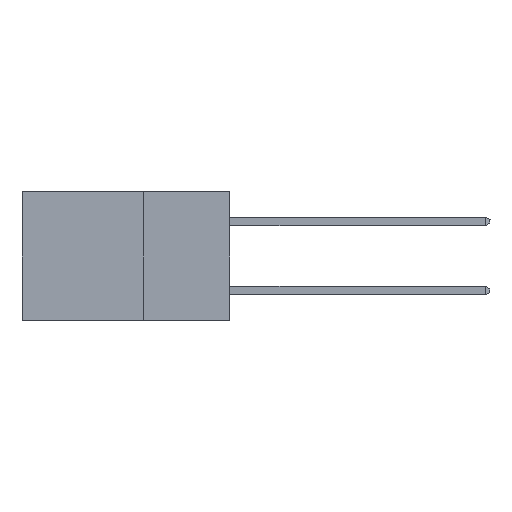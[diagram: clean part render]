
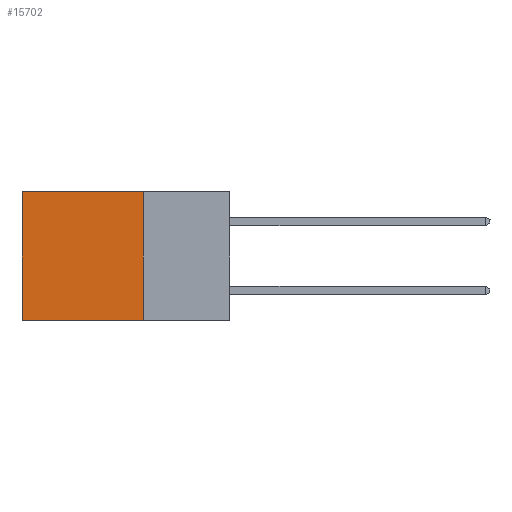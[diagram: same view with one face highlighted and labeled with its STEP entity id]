
A CAD part, left-side view. The second image highlights one B-rep face of the part: STEP entity #15702.
In plain terms, the highlighted planar face has unit normal (-1, 0, 0).
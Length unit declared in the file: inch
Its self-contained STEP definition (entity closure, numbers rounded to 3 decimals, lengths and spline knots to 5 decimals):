
#341 = DIRECTION ( 'NONE',  ( 0., 1., 0. ) ) ;
#380 = ORIENTED_EDGE ( 'NONE', *, *, #632, .T. ) ;
#448 = DIRECTION ( 'NONE',  ( 0., 0., -1. ) ) ;
#632 = EDGE_CURVE ( 'NONE', #5052, #20814, #19548, .T. ) ;
#1118 = DIRECTION ( 'NONE',  ( 0., 0., -1. ) ) ;
#2310 = CARTESIAN_POINT ( 'NONE',  ( 0.2615, 0.25, 0. ) ) ;
#2359 = VERTEX_POINT ( 'NONE', #10667 ) ;
#2882 = VECTOR ( 'NONE', #13404, 39.37008 ) ;
#5052 = VERTEX_POINT ( 'NONE', #2310 ) ;
#5128 = EDGE_CURVE ( 'NONE', #19683, #2359, #17520, .T. ) ;
#5238 = CARTESIAN_POINT ( 'NONE',  ( 0.2615, 0.25, -0.37 ) ) ;
#5542 = VECTOR ( 'NONE', #16861, 39.37008 ) ;
#7183 = CARTESIAN_POINT ( 'NONE',  ( 0.2615, 0.6, -0.37 ) ) ;
#7381 = EDGE_LOOP ( 'NONE', ( #21998, #22691, #16037, #380 ) ) ;
#8088 = CARTESIAN_POINT ( 'NONE',  ( 0.2615, 0.25, -0.37 ) ) ;
#8102 = DIRECTION ( 'NONE',  ( 1., 0., 0. ) ) ;
#10667 = CARTESIAN_POINT ( 'NONE',  ( 0.2615, 0.6, -0.37 ) ) ;
#11519 = EDGE_CURVE ( 'NONE', #20814, #2359, #20608, .T. ) ;
#12267 = VECTOR ( 'NONE', #1118, 39.37008 ) ;
#13404 = DIRECTION ( 'NONE',  ( 0., 1., 0. ) ) ;
#13490 = CARTESIAN_POINT ( 'NONE',  ( 0.2615, 0.6, 0. ) ) ;
#14147 = PLANE ( 'NONE',  #20635 ) ;
#14333 = LINE ( 'NONE', #20081, #12267 ) ;
#15417 = CARTESIAN_POINT ( 'NONE',  ( 0.2615, 0.25, 0. ) ) ;
#15702 = ADVANCED_FACE ( 'NONE', ( #17910 ), #14147, .F. ) ;
#16037 = ORIENTED_EDGE ( 'NONE', *, *, #16890, .F. ) ;
#16861 = DIRECTION ( 'NONE',  ( 0., 0., -1. ) ) ;
#16890 = EDGE_CURVE ( 'NONE', #5052, #19683, #14333, .T. ) ;
#17520 = LINE ( 'NONE', #8088, #2882 ) ;
#17789 = CARTESIAN_POINT ( 'NONE',  ( 0.2615, 0.25, -0.37 ) ) ;
#17910 = FACE_OUTER_BOUND ( 'NONE', #7381, .T. ) ;
#19023 = VECTOR ( 'NONE', #341, 39.37008 ) ;
#19548 = LINE ( 'NONE', #15417, #19023 ) ;
#19683 = VERTEX_POINT ( 'NONE', #5238 ) ;
#20081 = CARTESIAN_POINT ( 'NONE',  ( 0.2615, 0.25, -0.37 ) ) ;
#20608 = LINE ( 'NONE', #7183, #5542 ) ;
#20635 = AXIS2_PLACEMENT_3D ( 'NONE', #17789, #8102, #448 ) ;
#20814 = VERTEX_POINT ( 'NONE', #13490 ) ;
#21998 = ORIENTED_EDGE ( 'NONE', *, *, #11519, .T. ) ;
#22691 = ORIENTED_EDGE ( 'NONE', *, *, #5128, .F. ) ;
